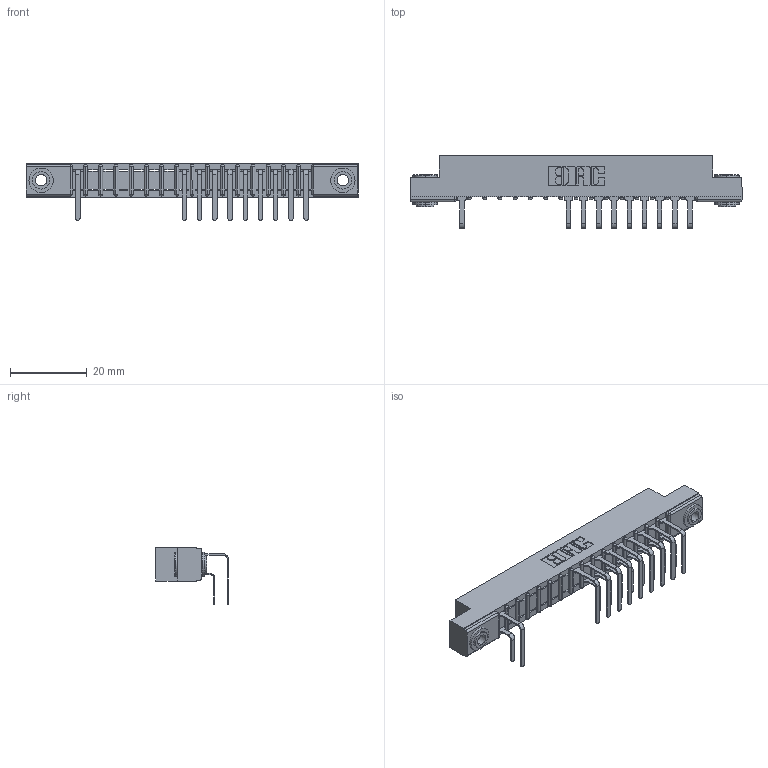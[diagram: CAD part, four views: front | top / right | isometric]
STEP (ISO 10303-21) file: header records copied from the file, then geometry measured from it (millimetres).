
FILE_DESCRIPTION (( 'STEP AP203' ), '1' );
FILE_NAME ('307-032-558-203.STEP', '2018-08-04T22:51:34', ( '' ), ( '' ), 'SwSTEP 2.0', 'SolidWorks 2016', '' );
FILE_SCHEMA (( 'CONFIG_CONTROL_DESIGN' ));
Length unit declared in the file: inch
Products named in the file (5): 345-250-002_345-250-002-102; 307-032-558-203; 307 Part_.156 Dia Mounting Holes; 307-290-001_558 559 - 1 (Single); 307-290-001_558 - 2 (Single)
Assembly tree (22 placements, depth 2):
  307-032-558-203
    307 Part_.156 Dia Mounting Holes
    307-290-001_558 559 - 1 (Single)  x9
    307-290-001_558 - 2 (Single)  x10
    345-250-002_345-250-002-102  x2
Bounding box: 86.41 x 18.96 x 14.81 mm (x, y, z)
Volume: 5571.7 mm3; surface area: 9265.6 mm2
Topology: 22 solids, 22 shells, 1267 faces, 3549 edges, 2290 vertices
Faces by surface type: plane 799, cylinder 426, sphere 34, cone 8
Entity records: 19530 total; most frequent: CARTESIAN_POINT 3242, ORIENTED_EDGE 3214, DIRECTION 3187, EDGE_CURVE 1607, LINE 1213, VECTOR 1213, VERTEX_POINT 1042, AXIS2_PLACEMENT_3D 987
